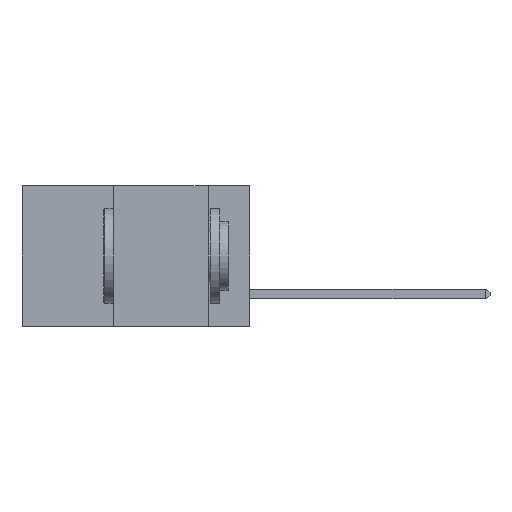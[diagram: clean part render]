
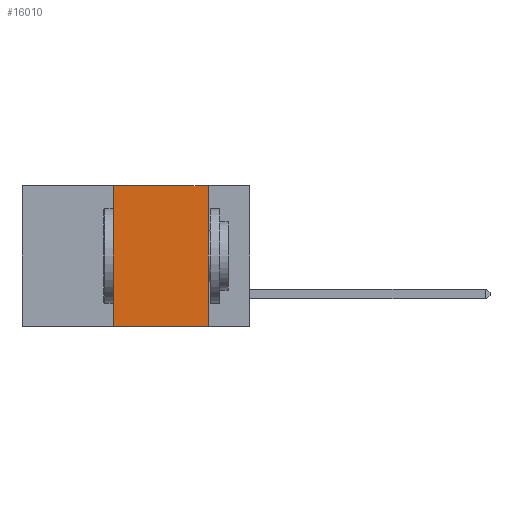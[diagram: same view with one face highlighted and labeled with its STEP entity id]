
A CAD part, left-side view. The second image highlights one B-rep face of the part: STEP entity #16010.
In plain terms, the highlighted planar face has unit normal (-1, 0, 0).
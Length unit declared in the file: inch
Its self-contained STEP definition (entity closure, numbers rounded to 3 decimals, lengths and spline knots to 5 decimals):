
#27 = VECTOR ( 'NONE', #26661, 39.37008 ) ;
#118 = CARTESIAN_POINT ( 'NONE',  ( 0., 0.11, -0.37 ) ) ;
#728 = ORIENTED_EDGE ( 'NONE', *, *, #30870, .T. ) ;
#757 = LINE ( 'NONE', #27394, #18462 ) ;
#2345 = ORIENTED_EDGE ( 'NONE', *, *, #11973, .F. ) ;
#2447 = DIRECTION ( 'NONE',  ( 1., 0., 0. ) ) ;
#4505 = CARTESIAN_POINT ( 'NONE',  ( 0., 0.6, -0.37 ) ) ;
#6971 = VERTEX_POINT ( 'NONE', #33016 ) ;
#7921 = DIRECTION ( 'NONE',  ( 0., -1., 0. ) ) ;
#8213 = EDGE_LOOP ( 'NONE', ( #18937, #2345, #20928, #728 ) ) ;
#9056 = LINE ( 'NONE', #4505, #17768 ) ;
#11973 = EDGE_CURVE ( 'NONE', #36415, #6971, #757, .T. ) ;
#15387 = FACE_OUTER_BOUND ( 'NONE', #8213, .T. ) ;
#15437 = CARTESIAN_POINT ( 'NONE',  ( 0., 0.36, 0. ) ) ;
#16010 = ADVANCED_FACE ( 'NONE', ( #15387 ), #18973, .F. ) ;
#17768 = VECTOR ( 'NONE', #30487, 39.37008 ) ;
#18462 = VECTOR ( 'NONE', #7921, 39.37008 ) ;
#18894 = EDGE_CURVE ( 'NONE', #38107, #36415, #37815, .T. ) ;
#18937 = ORIENTED_EDGE ( 'NONE', *, *, #21832, .F. ) ;
#18973 = PLANE ( 'NONE',  #23003 ) ;
#20928 = ORIENTED_EDGE ( 'NONE', *, *, #18894, .F. ) ;
#21832 = EDGE_CURVE ( 'NONE', #6971, #29531, #26342, .T. ) ;
#23003 = AXIS2_PLACEMENT_3D ( 'NONE', #40850, #2447, #25436 ) ;
#23401 = CARTESIAN_POINT ( 'NONE',  ( 0., 0.11, 0. ) ) ;
#25304 = CARTESIAN_POINT ( 'NONE',  ( 0., 0.36, -0.37 ) ) ;
#25436 = DIRECTION ( 'NONE',  ( 0., 0., -1. ) ) ;
#26342 = LINE ( 'NONE', #23401, #27 ) ;
#26661 = DIRECTION ( 'NONE',  ( 0., 0., -1. ) ) ;
#27394 = CARTESIAN_POINT ( 'NONE',  ( 0., 0.6, 0. ) ) ;
#27686 = VECTOR ( 'NONE', #40625, 39.37008 ) ;
#28253 = CARTESIAN_POINT ( 'NONE',  ( 0., 0.36, 0. ) ) ;
#29531 = VERTEX_POINT ( 'NONE', #118 ) ;
#30487 = DIRECTION ( 'NONE',  ( 0., -1., 0. ) ) ;
#30870 = EDGE_CURVE ( 'NONE', #38107, #29531, #9056, .T. ) ;
#33016 = CARTESIAN_POINT ( 'NONE',  ( 0., 0.11, 0. ) ) ;
#36415 = VERTEX_POINT ( 'NONE', #15437 ) ;
#37815 = LINE ( 'NONE', #28253, #27686 ) ;
#38107 = VERTEX_POINT ( 'NONE', #25304 ) ;
#40625 = DIRECTION ( 'NONE',  ( 0., 0., 1. ) ) ;
#40850 = CARTESIAN_POINT ( 'NONE',  ( 0., 0.6, 0. ) ) ;
